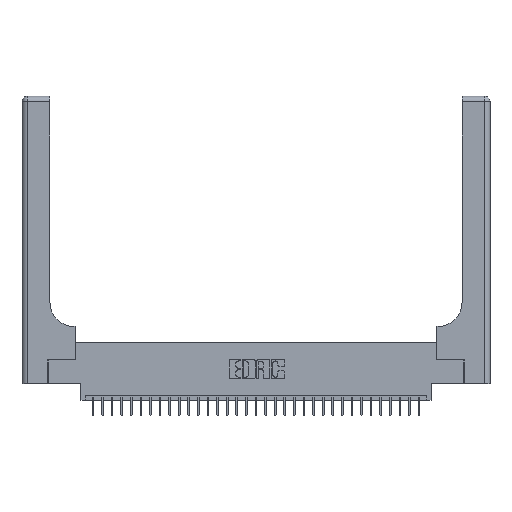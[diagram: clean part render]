
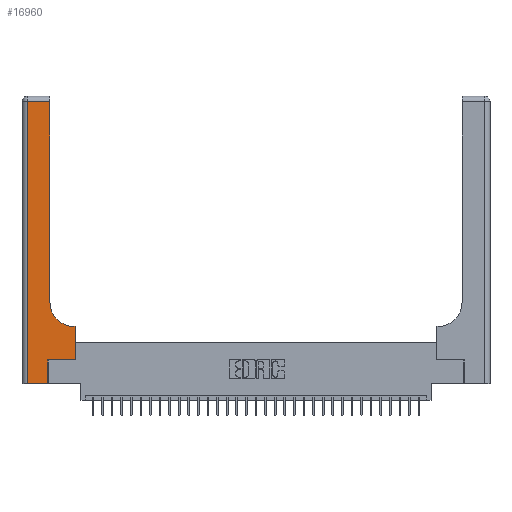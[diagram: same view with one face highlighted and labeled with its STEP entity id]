
A CAD part, top view. The second image highlights one B-rep face of the part: STEP entity #16960.
In plain terms, the highlighted planar face has unit normal (0, 0, 1).
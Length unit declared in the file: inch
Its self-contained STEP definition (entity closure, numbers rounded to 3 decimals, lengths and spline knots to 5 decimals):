
#571 = DIRECTION ( 'NONE',  ( 0., 1., 0. ) ) ;
#1512 = DIRECTION ( 'NONE',  ( 0., 0., -1. ) ) ;
#1752 = EDGE_CURVE ( 'NONE', #31716, #32579, #14418, .T. ) ;
#1889 = EDGE_CURVE ( 'NONE', #28587, #10529, #17274, .T. ) ;
#2673 = DIRECTION ( 'NONE',  ( 0., -1., 0. ) ) ;
#2679 = CARTESIAN_POINT ( 'NONE',  ( 0.2915, 3., 0.37 ) ) ;
#3944 = EDGE_CURVE ( 'NONE', #32579, #28587, #31295, .T. ) ;
#4626 = CARTESIAN_POINT ( 'NONE',  ( 0.06, 0., 0.37 ) ) ;
#4852 = CARTESIAN_POINT ( 'NONE',  ( 0., 0., 0.37 ) ) ;
#5253 = VECTOR ( 'NONE', #20975, 39.37008 ) ;
#5837 = LINE ( 'NONE', #21756, #18940 ) ;
#6047 = CARTESIAN_POINT ( 'NONE',  ( 0.269, 0.25, 0.37 ) ) ;
#6534 = CARTESIAN_POINT ( 'NONE',  ( 0.06, 2.94, 0.37 ) ) ;
#8038 = ORIENTED_EDGE ( 'NONE', *, *, #27517, .T. ) ;
#8118 = EDGE_CURVE ( 'NONE', #30077, #31716, #20474, .T. ) ;
#8138 = CARTESIAN_POINT ( 'NONE',  ( 0.2915, 0.6, 0.37 ) ) ;
#8794 = DIRECTION ( 'NONE',  ( 1., 0., 0. ) ) ;
#9473 = VECTOR ( 'NONE', #571, 39.37008 ) ;
#9743 = VECTOR ( 'NONE', #10122, 39.37008 ) ;
#10122 = DIRECTION ( 'NONE',  ( 1., 0., 0. ) ) ;
#10529 = VERTEX_POINT ( 'NONE', #6047 ) ;
#10758 = DIRECTION ( 'NONE',  ( -1., 0., 0. ) ) ;
#11145 = CARTESIAN_POINT ( 'NONE',  ( 0.269, 0., 0.37 ) ) ;
#11575 = VECTOR ( 'NONE', #10758, 39.37008 ) ;
#11585 = ORIENTED_EDGE ( 'NONE', *, *, #25985, .T. ) ;
#11762 = CARTESIAN_POINT ( 'NONE',  ( 0.5415, 0.6, 0.37 ) ) ;
#12492 = CARTESIAN_POINT ( 'NONE',  ( 0.269, 0., 0.37 ) ) ;
#12611 = ORIENTED_EDGE ( 'NONE', *, *, #8118, .T. ) ;
#13182 = FACE_OUTER_BOUND ( 'NONE', #27861, .T. ) ;
#13680 = DIRECTION ( 'NONE',  ( 0., 1., 0. ) ) ;
#14418 = LINE ( 'NONE', #26042, #19689 ) ;
#14626 = PLANE ( 'NONE',  #16672 ) ;
#14873 = VERTEX_POINT ( 'NONE', #23318 ) ;
#15683 = CARTESIAN_POINT ( 'NONE',  ( 0.5415, 0.85, 0.37 ) ) ;
#16159 = EDGE_CURVE ( 'NONE', #14873, #19025, #24583, .T. ) ;
#16563 = EDGE_CURVE ( 'NONE', #19025, #19328, #25364, .T. ) ;
#16672 = AXIS2_PLACEMENT_3D ( 'NONE', #32769, #1512, #19846 ) ;
#16960 = ADVANCED_FACE ( 'NONE', ( #13182 ), #14626, .F. ) ;
#16986 = ORIENTED_EDGE ( 'NONE', *, *, #16159, .T. ) ;
#17274 = LINE ( 'NONE', #11145, #9473 ) ;
#17605 = LINE ( 'NONE', #29176, #24446 ) ;
#18299 = DIRECTION ( 'NONE',  ( 1., 0., 0. ) ) ;
#18577 = ORIENTED_EDGE ( 'NONE', *, *, #29553, .T. ) ;
#18763 = ORIENTED_EDGE ( 'NONE', *, *, #1752, .T. ) ;
#18940 = VECTOR ( 'NONE', #8794, 39.37008 ) ;
#19025 = VERTEX_POINT ( 'NONE', #11762 ) ;
#19328 = VERTEX_POINT ( 'NONE', #26280 ) ;
#19689 = VECTOR ( 'NONE', #2673, 39.37008 ) ;
#19846 = DIRECTION ( 'NONE',  ( -1., 0., 0. ) ) ;
#20474 = LINE ( 'NONE', #30301, #26543 ) ;
#20975 = DIRECTION ( 'NONE',  ( 0., 1., 0. ) ) ;
#21756 = CARTESIAN_POINT ( 'NONE',  ( 0.269, 0.25, 0.37 ) ) ;
#23024 = CARTESIAN_POINT ( 'NONE',  ( 0.2915, 2.94, 0.37 ) ) ;
#23318 = CARTESIAN_POINT ( 'NONE',  ( 0.5585, 0.6, 0.37 ) ) ;
#24446 = VECTOR ( 'NONE', #13680, 39.37008 ) ;
#24583 = LINE ( 'NONE', #8138, #11575 ) ;
#25364 = CIRCLE ( 'NONE', #33577, 0.25 ) ;
#25985 = EDGE_CURVE ( 'NONE', #29675, #14873, #17605, .T. ) ;
#26042 = CARTESIAN_POINT ( 'NONE',  ( 0.06, 3., 0.37 ) ) ;
#26280 = CARTESIAN_POINT ( 'NONE',  ( 0.2915, 0.85, 0.37 ) ) ;
#26543 = VECTOR ( 'NONE', #32921, 39.37008 ) ;
#27497 = CARTESIAN_POINT ( 'NONE',  ( 0.5585, 0.25, 0.37 ) ) ;
#27517 = EDGE_CURVE ( 'NONE', #19328, #30077, #32134, .T. ) ;
#27861 = EDGE_LOOP ( 'NONE', ( #8038, #12611, #18763, #31950, #33809, #18577, #11585, #16986, #32539 ) ) ;
#28587 = VERTEX_POINT ( 'NONE', #12492 ) ;
#29176 = CARTESIAN_POINT ( 'NONE',  ( 0.5585, 0.25, 0.37 ) ) ;
#29553 = EDGE_CURVE ( 'NONE', #10529, #29675, #5837, .T. ) ;
#29675 = VERTEX_POINT ( 'NONE', #27497 ) ;
#30077 = VERTEX_POINT ( 'NONE', #23024 ) ;
#30301 = CARTESIAN_POINT ( 'NONE',  ( 0., 2.94, 0.37 ) ) ;
#31295 = LINE ( 'NONE', #4852, #9743 ) ;
#31716 = VERTEX_POINT ( 'NONE', #6534 ) ;
#31950 = ORIENTED_EDGE ( 'NONE', *, *, #3944, .T. ) ;
#32134 = LINE ( 'NONE', #2679, #5253 ) ;
#32539 = ORIENTED_EDGE ( 'NONE', *, *, #16563, .T. ) ;
#32579 = VERTEX_POINT ( 'NONE', #4626 ) ;
#32769 = CARTESIAN_POINT ( 'NONE',  ( 0., 3., 0.37 ) ) ;
#32921 = DIRECTION ( 'NONE',  ( -1., 0., 0. ) ) ;
#33577 = AXIS2_PLACEMENT_3D ( 'NONE', #15683, #33803, #18299 ) ;
#33803 = DIRECTION ( 'NONE',  ( 0., 0., -1. ) ) ;
#33809 = ORIENTED_EDGE ( 'NONE', *, *, #1889, .T. ) ;
